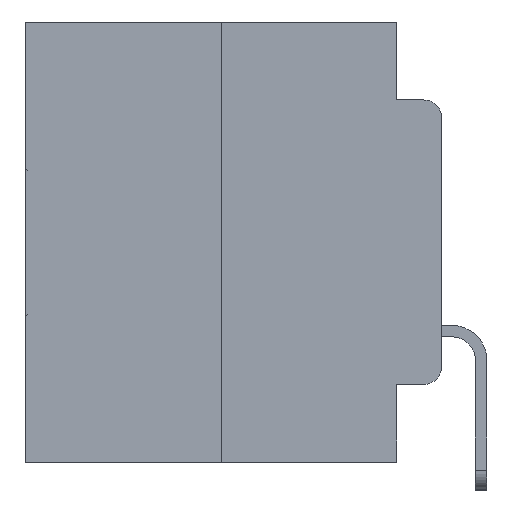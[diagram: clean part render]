
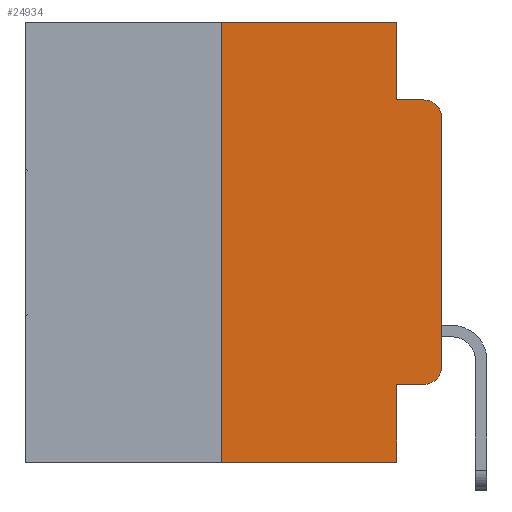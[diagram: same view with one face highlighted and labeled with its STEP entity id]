
A CAD part, left-side view. The second image highlights one B-rep face of the part: STEP entity #24934.
In plain terms, the highlighted planar face has unit normal (-1, 0, 0).
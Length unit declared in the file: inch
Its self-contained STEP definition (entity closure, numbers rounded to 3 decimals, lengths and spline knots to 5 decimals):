
#285 = CARTESIAN_POINT ( 'NONE',  ( 0., 0.25, 0. ) ) ;
#336 = ORIENTED_EDGE ( 'NONE', *, *, #23123, .T. ) ;
#473 = ORIENTED_EDGE ( 'NONE', *, *, #20138, .T. ) ;
#476 = CARTESIAN_POINT ( 'NONE',  ( 0., 0.051, 0. ) ) ;
#498 = CARTESIAN_POINT ( 'NONE',  ( 0., 0.02, -0.3915 ) ) ;
#1287 = EDGE_CURVE ( 'NONE', #22138, #27689, #25137, .T. ) ;
#1316 = CARTESIAN_POINT ( 'NONE',  ( 0., 0.473, 0. ) ) ;
#1398 = VECTOR ( 'NONE', #2798, 39.37008 ) ;
#1647 = LINE ( 'NONE', #15065, #24985 ) ;
#1695 = CARTESIAN_POINT ( 'NONE',  ( 0., 0.051, 0. ) ) ;
#2028 = ORIENTED_EDGE ( 'NONE', *, *, #27556, .F. ) ;
#2195 = ORIENTED_EDGE ( 'NONE', *, *, #19924, .F. ) ;
#2798 = DIRECTION ( 'NONE',  ( 0., 0., -1. ) ) ;
#2818 = DIRECTION ( 'NONE',  ( 0., 0., -1. ) ) ;
#2838 = EDGE_CURVE ( 'NONE', #27689, #24032, #29181, .T. ) ;
#3115 = VERTEX_POINT ( 'NONE', #28426 ) ;
#3153 = AXIS2_PLACEMENT_3D ( 'NONE', #1316, #17270, #3649 ) ;
#3649 = DIRECTION ( 'NONE',  ( 0., 0., -1. ) ) ;
#4382 = CIRCLE ( 'NONE', #18808, 0.02 ) ;
#5620 = CARTESIAN_POINT ( 'NONE',  ( 0., 0.02, -0.1085 ) ) ;
#5696 = VECTOR ( 'NONE', #16221, 39.37008 ) ;
#5945 = VERTEX_POINT ( 'NONE', #27325 ) ;
#6689 = ORIENTED_EDGE ( 'NONE', *, *, #26041, .F. ) ;
#7135 = ORIENTED_EDGE ( 'NONE', *, *, #1287, .F. ) ;
#7260 = VECTOR ( 'NONE', #11327, 39.37008 ) ;
#7505 = EDGE_CURVE ( 'NONE', #20296, #24032, #4382, .T. ) ;
#7511 = ORIENTED_EDGE ( 'NONE', *, *, #18648, .T. ) ;
#7541 = ORIENTED_EDGE ( 'NONE', *, *, #2838, .F. ) ;
#7924 = DIRECTION ( 'NONE',  ( 0., 0., -1. ) ) ;
#8079 = VERTEX_POINT ( 'NONE', #19457 ) ;
#8473 = FACE_OUTER_BOUND ( 'NONE', #18240, .T. ) ;
#9521 = VECTOR ( 'NONE', #10352, 39.37008 ) ;
#10176 = AXIS2_PLACEMENT_3D ( 'NONE', #498, #16488, #2818 ) ;
#10352 = DIRECTION ( 'NONE',  ( 0., 0., 1. ) ) ;
#11171 = CARTESIAN_POINT ( 'NONE',  ( 0., 0.473, 0. ) ) ;
#11327 = DIRECTION ( 'NONE',  ( 0., 0., -1. ) ) ;
#11398 = VECTOR ( 'NONE', #19056, 39.37008 ) ;
#12043 = EDGE_CURVE ( 'NONE', #20127, #20296, #22843, .T. ) ;
#12427 = LINE ( 'NONE', #27477, #5696 ) ;
#12802 = VECTOR ( 'NONE', #13647, 39.37008 ) ;
#13401 = DIRECTION ( 'NONE',  ( 0., -1., 0. ) ) ;
#13647 = DIRECTION ( 'NONE',  ( 0., -1., 0. ) ) ;
#14115 = CARTESIAN_POINT ( 'NONE',  ( 0., 0.051, -0.4115 ) ) ;
#15065 = CARTESIAN_POINT ( 'NONE',  ( 0., 0.25, 0. ) ) ;
#15226 = ORIENTED_EDGE ( 'NONE', *, *, #7505, .T. ) ;
#16221 = DIRECTION ( 'NONE',  ( 0., -1., 0. ) ) ;
#16396 = CARTESIAN_POINT ( 'NONE',  ( 0., 0., -0.3915 ) ) ;
#16488 = DIRECTION ( 'NONE',  ( -1., 0., 0. ) ) ;
#16831 = CARTESIAN_POINT ( 'NONE',  ( 0., 0.051, -0.0885 ) ) ;
#17179 = PLANE ( 'NONE',  #3153 ) ;
#17270 = DIRECTION ( 'NONE',  ( 1., 0., 0. ) ) ;
#17913 = CARTESIAN_POINT ( 'NONE',  ( 0., 0.051, -0.0885 ) ) ;
#18122 = CARTESIAN_POINT ( 'NONE',  ( 0., 0.051, 0. ) ) ;
#18240 = EDGE_LOOP ( 'NONE', ( #23418, #15226, #7541, #7135, #2195, #2028, #7511, #6689, #336, #473 ) ) ;
#18648 = EDGE_CURVE ( 'NONE', #8079, #5945, #19480, .T. ) ;
#18808 = AXIS2_PLACEMENT_3D ( 'NONE', #5620, #21377, #7924 ) ;
#19056 = DIRECTION ( 'NONE',  ( 0., -1., 0. ) ) ;
#19457 = CARTESIAN_POINT ( 'NONE',  ( 0., 0.25, -0.5 ) ) ;
#19478 = VERTEX_POINT ( 'NONE', #14115 ) ;
#19480 = LINE ( 'NONE', #24875, #12802 ) ;
#19526 = LINE ( 'NONE', #476, #1398 ) ;
#19924 = EDGE_CURVE ( 'NONE', #25995, #22138, #27567, .T. ) ;
#20127 = VERTEX_POINT ( 'NONE', #16396 ) ;
#20138 = EDGE_CURVE ( 'NONE', #3115, #20127, #25793, .T. ) ;
#20296 = VERTEX_POINT ( 'NONE', #25765 ) ;
#21377 = DIRECTION ( 'NONE',  ( -1., 0., 0. ) ) ;
#22138 = VERTEX_POINT ( 'NONE', #1695 ) ;
#22843 = LINE ( 'NONE', #23768, #9521 ) ;
#23123 = EDGE_CURVE ( 'NONE', #19478, #3115, #12427, .T. ) ;
#23418 = ORIENTED_EDGE ( 'NONE', *, *, #12043, .T. ) ;
#23768 = CARTESIAN_POINT ( 'NONE',  ( 0., 0., 0. ) ) ;
#24032 = VERTEX_POINT ( 'NONE', #27299 ) ;
#24875 = CARTESIAN_POINT ( 'NONE',  ( 0., 0.473, -0.5 ) ) ;
#24934 = ADVANCED_FACE ( 'NONE', ( #8473 ), #17179, .F. ) ;
#24985 = VECTOR ( 'NONE', #26225, 39.37008 ) ;
#25137 = LINE ( 'NONE', #18122, #7260 ) ;
#25765 = CARTESIAN_POINT ( 'NONE',  ( 0., 0., -0.1085 ) ) ;
#25793 = CIRCLE ( 'NONE', #10176, 0.02 ) ;
#25995 = VERTEX_POINT ( 'NONE', #285 ) ;
#26041 = EDGE_CURVE ( 'NONE', #19478, #5945, #19526, .T. ) ;
#26152 = VECTOR ( 'NONE', #13401, 39.37008 ) ;
#26225 = DIRECTION ( 'NONE',  ( 0., 0., 1. ) ) ;
#27299 = CARTESIAN_POINT ( 'NONE',  ( 0., 0.02, -0.0885 ) ) ;
#27325 = CARTESIAN_POINT ( 'NONE',  ( 0., 0.051, -0.5 ) ) ;
#27477 = CARTESIAN_POINT ( 'NONE',  ( 0., 0.051, -0.4115 ) ) ;
#27556 = EDGE_CURVE ( 'NONE', #8079, #25995, #1647, .T. ) ;
#27567 = LINE ( 'NONE', #11171, #26152 ) ;
#27689 = VERTEX_POINT ( 'NONE', #17913 ) ;
#28426 = CARTESIAN_POINT ( 'NONE',  ( 0., 0.02, -0.4115 ) ) ;
#29181 = LINE ( 'NONE', #16831, #11398 ) ;
